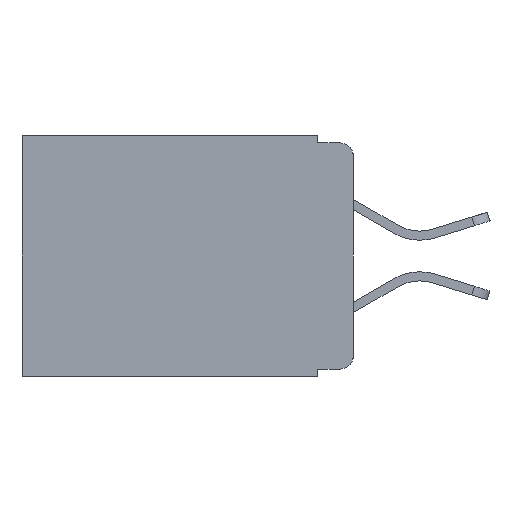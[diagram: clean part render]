
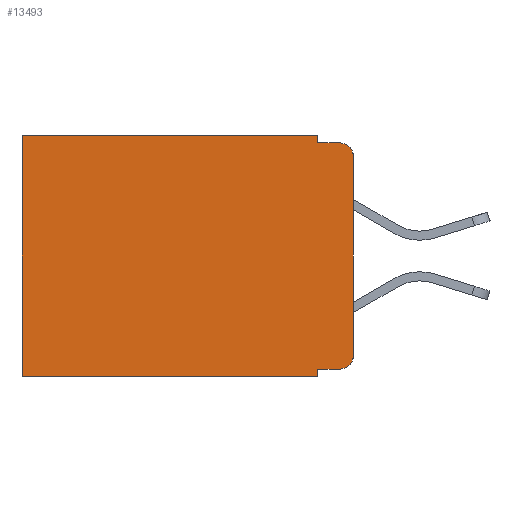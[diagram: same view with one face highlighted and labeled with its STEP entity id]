
A CAD part, left-side view. The second image highlights one B-rep face of the part: STEP entity #13493.
In plain terms, the highlighted planar face has unit normal (-1, 0, 0).
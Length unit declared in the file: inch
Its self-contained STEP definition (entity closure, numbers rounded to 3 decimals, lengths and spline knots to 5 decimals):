
#279 = DIRECTION ( 'NONE',  ( 0., 0., -1. ) ) ;
#478 = VERTEX_POINT ( 'NONE', #7574 ) ;
#845 = DIRECTION ( 'NONE',  ( 0., 0., -1. ) ) ;
#983 = DIRECTION ( 'NONE',  ( 0., 1., 0. ) ) ;
#1385 = EDGE_CURVE ( 'NONE', #14983, #3997, #15528, .T. ) ;
#1452 = CARTESIAN_POINT ( 'NONE',  ( 0.298, 0.051, 0. ) ) ;
#1676 = EDGE_LOOP ( 'NONE', ( #20338, #4862, #13232, #6110, #2283, #3918, #19404, #2312, #11447, #3071 ) ) ;
#1688 = EDGE_CURVE ( 'NONE', #17540, #5283, #15807, .T. ) ;
#1721 = VECTOR ( 'NONE', #6047, 39.37008 ) ;
#1808 = EDGE_CURVE ( 'NONE', #19772, #5283, #10856, .T. ) ;
#2283 = ORIENTED_EDGE ( 'NONE', *, *, #5405, .T. ) ;
#2312 = ORIENTED_EDGE ( 'NONE', *, *, #10290, .F. ) ;
#2323 = EDGE_CURVE ( 'NONE', #478, #24759, #10198, .T. ) ;
#2639 = VECTOR ( 'NONE', #5032, 39.37008 ) ;
#2998 = CARTESIAN_POINT ( 'NONE',  ( 0.298, 0., 0. ) ) ;
#3071 = ORIENTED_EDGE ( 'NONE', *, *, #22509, .T. ) ;
#3535 = CARTESIAN_POINT ( 'NONE',  ( 0.298, 0.02, -0.01 ) ) ;
#3812 = DIRECTION ( 'NONE',  ( 0., -1., 0. ) ) ;
#3918 = ORIENTED_EDGE ( 'NONE', *, *, #1688, .T. ) ;
#3997 = VERTEX_POINT ( 'NONE', #3535 ) ;
#4800 = CARTESIAN_POINT ( 'NONE',  ( 0.298, 0.473, 0. ) ) ;
#4862 = ORIENTED_EDGE ( 'NONE', *, *, #10684, .T. ) ;
#5032 = DIRECTION ( 'NONE',  ( 0., 0., -1. ) ) ;
#5048 = VECTOR ( 'NONE', #3812, 39.37008 ) ;
#5113 = VERTEX_POINT ( 'NONE', #1452 ) ;
#5283 = VERTEX_POINT ( 'NONE', #9423 ) ;
#5405 = EDGE_CURVE ( 'NONE', #5113, #17540, #14289, .T. ) ;
#6047 = DIRECTION ( 'NONE',  ( 0., 0., -1. ) ) ;
#6083 = PLANE ( 'NONE',  #12519 ) ;
#6110 = ORIENTED_EDGE ( 'NONE', *, *, #20634, .F. ) ;
#6578 = AXIS2_PLACEMENT_3D ( 'NONE', #23688, #12180, #279 ) ;
#7047 = LINE ( 'NONE', #21643, #1721 ) ;
#7574 = CARTESIAN_POINT ( 'NONE',  ( 0.298, 0.051, -0.333 ) ) ;
#7676 = CARTESIAN_POINT ( 'NONE',  ( 0.298, 0.051, -0.01 ) ) ;
#8028 = DIRECTION ( 'NONE',  ( 1., 0., 0. ) ) ;
#8059 = FACE_OUTER_BOUND ( 'NONE', #1676, .T. ) ;
#8550 = CARTESIAN_POINT ( 'NONE',  ( 0.298, 0.051, 0. ) ) ;
#8585 = DIRECTION ( 'NONE',  ( 0., 1., 0. ) ) ;
#9423 = CARTESIAN_POINT ( 'NONE',  ( 0.298, 0.473, -0.343 ) ) ;
#9574 = VECTOR ( 'NONE', #17300, 39.37008 ) ;
#9666 = CARTESIAN_POINT ( 'NONE',  ( 0.298, 0.051, -0.333 ) ) ;
#9973 = CARTESIAN_POINT ( 'NONE',  ( 0.298, 0.051, -0.343 ) ) ;
#10129 = CARTESIAN_POINT ( 'NONE',  ( 0.298, 0., -0.03 ) ) ;
#10198 = LINE ( 'NONE', #9666, #9574 ) ;
#10290 = EDGE_CURVE ( 'NONE', #478, #19772, #7047, .T. ) ;
#10342 = VERTEX_POINT ( 'NONE', #10129 ) ;
#10540 = DIRECTION ( 'NONE',  ( 0., 0., -1. ) ) ;
#10684 = EDGE_CURVE ( 'NONE', #10342, #3997, #19269, .T. ) ;
#10856 = LINE ( 'NONE', #23029, #16102 ) ;
#11447 = ORIENTED_EDGE ( 'NONE', *, *, #2323, .T. ) ;
#11503 = CARTESIAN_POINT ( 'NONE',  ( 0.298, 0., 0. ) ) ;
#12180 = DIRECTION ( 'NONE',  ( -1., 0., 0. ) ) ;
#12519 = AXIS2_PLACEMENT_3D ( 'NONE', #19757, #8028, #21682 ) ;
#12730 = DIRECTION ( 'NONE',  ( -1., 0., 0. ) ) ;
#13179 = LINE ( 'NONE', #2998, #2639 ) ;
#13232 = ORIENTED_EDGE ( 'NONE', *, *, #1385, .F. ) ;
#13493 = ADVANCED_FACE ( 'NONE', ( #8059 ), #6083, .F. ) ;
#13879 = LINE ( 'NONE', #8550, #25219 ) ;
#14289 = LINE ( 'NONE', #11503, #23866 ) ;
#14895 = AXIS2_PLACEMENT_3D ( 'NONE', #24221, #12730, #845 ) ;
#14983 = VERTEX_POINT ( 'NONE', #22366 ) ;
#15528 = LINE ( 'NONE', #7676, #5048 ) ;
#15807 = LINE ( 'NONE', #4800, #23552 ) ;
#16102 = VECTOR ( 'NONE', #8585, 39.37008 ) ;
#17300 = DIRECTION ( 'NONE',  ( 0., -1., 0. ) ) ;
#17540 = VERTEX_POINT ( 'NONE', #22866 ) ;
#19103 = DIRECTION ( 'NONE',  ( 0., 0., -1. ) ) ;
#19269 = CIRCLE ( 'NONE', #14895, 0.02 ) ;
#19404 = ORIENTED_EDGE ( 'NONE', *, *, #1808, .F. ) ;
#19757 = CARTESIAN_POINT ( 'NONE',  ( 0.298, 0., 0. ) ) ;
#19772 = VERTEX_POINT ( 'NONE', #9973 ) ;
#19873 = CIRCLE ( 'NONE', #6578, 0.02 ) ;
#20338 = ORIENTED_EDGE ( 'NONE', *, *, #22724, .F. ) ;
#20634 = EDGE_CURVE ( 'NONE', #5113, #14983, #13879, .T. ) ;
#21224 = VERTEX_POINT ( 'NONE', #22715 ) ;
#21643 = CARTESIAN_POINT ( 'NONE',  ( 0.298, 0.051, 0. ) ) ;
#21682 = DIRECTION ( 'NONE',  ( 0., 0., -1. ) ) ;
#22366 = CARTESIAN_POINT ( 'NONE',  ( 0.298, 0.051, -0.01 ) ) ;
#22509 = EDGE_CURVE ( 'NONE', #24759, #21224, #19873, .T. ) ;
#22715 = CARTESIAN_POINT ( 'NONE',  ( 0.298, 0., -0.313 ) ) ;
#22724 = EDGE_CURVE ( 'NONE', #10342, #21224, #13179, .T. ) ;
#22866 = CARTESIAN_POINT ( 'NONE',  ( 0.298, 0.473, 0. ) ) ;
#23029 = CARTESIAN_POINT ( 'NONE',  ( 0.298, 0., -0.343 ) ) ;
#23552 = VECTOR ( 'NONE', #19103, 39.37008 ) ;
#23688 = CARTESIAN_POINT ( 'NONE',  ( 0.298, 0.02, -0.313 ) ) ;
#23866 = VECTOR ( 'NONE', #983, 39.37008 ) ;
#24221 = CARTESIAN_POINT ( 'NONE',  ( 0.298, 0.02, -0.03 ) ) ;
#24759 = VERTEX_POINT ( 'NONE', #25238 ) ;
#25219 = VECTOR ( 'NONE', #10540, 39.37008 ) ;
#25238 = CARTESIAN_POINT ( 'NONE',  ( 0.298, 0.02, -0.333 ) ) ;
